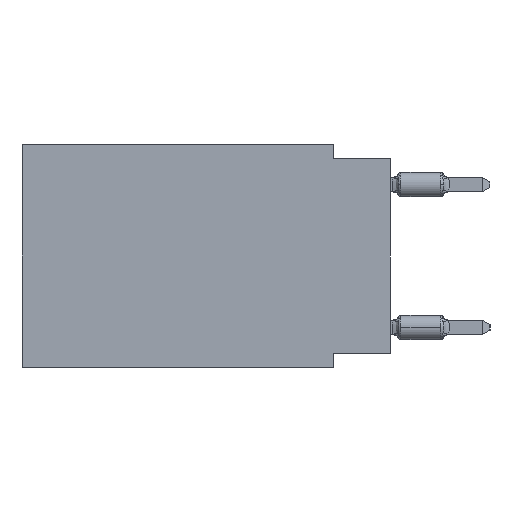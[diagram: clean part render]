
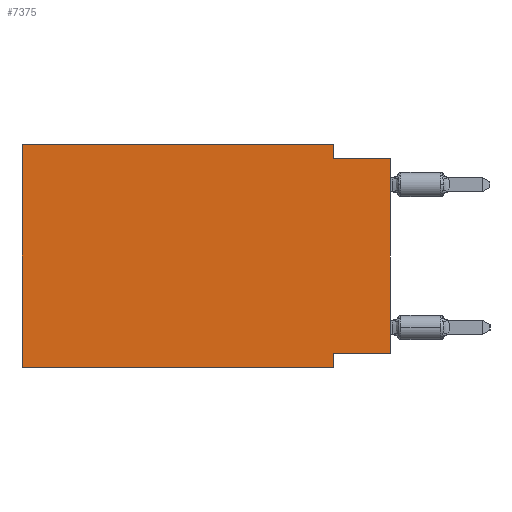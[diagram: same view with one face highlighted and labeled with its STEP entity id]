
A CAD part, left-side view. The second image highlights one B-rep face of the part: STEP entity #7375.
In plain terms, the highlighted planar face has unit normal (-1, 0, 0).
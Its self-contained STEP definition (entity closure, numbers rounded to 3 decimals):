
#169 = CARTESIAN_POINT ( 'NONE',  ( 0., 2.54, 0. ) ) ;
#2440 = ORIENTED_EDGE ( 'NONE', *, *, #37005, .T. ) ;
#3005 = VERTEX_POINT ( 'NONE', #38410 ) ;
#3457 = LINE ( 'NONE', #36537, #50990 ) ;
#3582 = LINE ( 'NONE', #32862, #7702 ) ;
#3731 = VECTOR ( 'NONE', #11823, 1000. ) ;
#4419 = VECTOR ( 'NONE', #9412, 1000. ) ;
#6550 = DIRECTION ( 'NONE',  ( 0., 0., 1. ) ) ;
#6747 = CARTESIAN_POINT ( 'NONE',  ( 0., 16.383, 0. ) ) ;
#7021 = ORIENTED_EDGE ( 'NONE', *, *, #34202, .T. ) ;
#7237 = DIRECTION ( 'NONE',  ( 0., -1., 0. ) ) ;
#7350 = CARTESIAN_POINT ( 'NONE',  ( 0., 16.383, 0. ) ) ;
#7375 = ADVANCED_FACE ( 'NONE', ( #44193 ), #24103, .F. ) ;
#7702 = VECTOR ( 'NONE', #44276, 1000. ) ;
#7764 = EDGE_CURVE ( 'NONE', #28013, #42736, #15905, .T. ) ;
#8222 = CARTESIAN_POINT ( 'NONE',  ( 0., 0., -9.271 ) ) ;
#9412 = DIRECTION ( 'NONE',  ( 0., -1., 0. ) ) ;
#10218 = CARTESIAN_POINT ( 'NONE',  ( 0., 2.54, -9.271 ) ) ;
#11292 = CARTESIAN_POINT ( 'NONE',  ( 0., 16.383, 0. ) ) ;
#11357 = DIRECTION ( 'NONE',  ( 0., 0., -1. ) ) ;
#11823 = DIRECTION ( 'NONE',  ( 0., -1., 0. ) ) ;
#14249 = LINE ( 'NONE', #37858, #24357 ) ;
#15905 = LINE ( 'NONE', #11292, #3731 ) ;
#16024 = EDGE_CURVE ( 'NONE', #24890, #28013, #16033, .T. ) ;
#16033 = LINE ( 'NONE', #7350, #24914 ) ;
#17414 = ORIENTED_EDGE ( 'NONE', *, *, #48316, .F. ) ;
#19610 = EDGE_CURVE ( 'NONE', #3005, #48276, #41993, .T. ) ;
#20754 = LINE ( 'NONE', #169, #43740 ) ;
#21306 = DIRECTION ( 'NONE',  ( 0., 1., 0. ) ) ;
#23754 = ORIENTED_EDGE ( 'NONE', *, *, #16024, .F. ) ;
#24103 = PLANE ( 'NONE',  #35739 ) ;
#24357 = VECTOR ( 'NONE', #21306, 1000. ) ;
#24890 = VERTEX_POINT ( 'NONE', #26294 ) ;
#24914 = VECTOR ( 'NONE', #6550, 1000. ) ;
#25377 = VERTEX_POINT ( 'NONE', #10218 ) ;
#26294 = CARTESIAN_POINT ( 'NONE',  ( 0., 16.383, -9.906 ) ) ;
#26539 = DIRECTION ( 'NONE',  ( 0., 0., 1. ) ) ;
#28013 = VERTEX_POINT ( 'NONE', #35635 ) ;
#29363 = VERTEX_POINT ( 'NONE', #8222 ) ;
#29427 = ORIENTED_EDGE ( 'NONE', *, *, #19610, .F. ) ;
#30350 = ORIENTED_EDGE ( 'NONE', *, *, #53325, .F. ) ;
#30877 = CARTESIAN_POINT ( 'NONE',  ( 0., 0., 0. ) ) ;
#32862 = CARTESIAN_POINT ( 'NONE',  ( 0., 2.54, -9.906 ) ) ;
#33227 = DIRECTION ( 'NONE',  ( 0., 0., -1. ) ) ;
#34202 = EDGE_CURVE ( 'NONE', #24890, #43339, #3457, .T. ) ;
#34960 = LINE ( 'NONE', #30877, #52023 ) ;
#35383 = EDGE_LOOP ( 'NONE', ( #2440, #29427, #17414, #42789, #23754, #7021, #30350, #47839 ) ) ;
#35635 = CARTESIAN_POINT ( 'NONE',  ( 0., 16.383, 0. ) ) ;
#35739 = AXIS2_PLACEMENT_3D ( 'NONE', #6747, #43925, #11357 ) ;
#36537 = CARTESIAN_POINT ( 'NONE',  ( 0., 16.383, -9.906 ) ) ;
#37005 = EDGE_CURVE ( 'NONE', #29363, #48276, #34960, .T. ) ;
#37018 = CARTESIAN_POINT ( 'NONE',  ( 0., 2.54, -9.906 ) ) ;
#37477 = CARTESIAN_POINT ( 'NONE',  ( 0., 2.54, 0. ) ) ;
#37858 = CARTESIAN_POINT ( 'NONE',  ( 0., 0., -9.271 ) ) ;
#37996 = EDGE_CURVE ( 'NONE', #29363, #25377, #14249, .T. ) ;
#38410 = CARTESIAN_POINT ( 'NONE',  ( 0., 2.54, -0.635 ) ) ;
#41993 = LINE ( 'NONE', #43062, #4419 ) ;
#42736 = VERTEX_POINT ( 'NONE', #37477 ) ;
#42789 = ORIENTED_EDGE ( 'NONE', *, *, #7764, .F. ) ;
#43062 = CARTESIAN_POINT ( 'NONE',  ( 0., 0., -0.635 ) ) ;
#43339 = VERTEX_POINT ( 'NONE', #37018 ) ;
#43740 = VECTOR ( 'NONE', #33227, 1000. ) ;
#43925 = DIRECTION ( 'NONE',  ( 1., 0., 0. ) ) ;
#44193 = FACE_OUTER_BOUND ( 'NONE', #35383, .T. ) ;
#44276 = DIRECTION ( 'NONE',  ( 0., 0., -1. ) ) ;
#45185 = CARTESIAN_POINT ( 'NONE',  ( 0., 0., -0.635 ) ) ;
#47839 = ORIENTED_EDGE ( 'NONE', *, *, #37996, .F. ) ;
#48276 = VERTEX_POINT ( 'NONE', #45185 ) ;
#48316 = EDGE_CURVE ( 'NONE', #42736, #3005, #20754, .T. ) ;
#50990 = VECTOR ( 'NONE', #7237, 1000. ) ;
#52023 = VECTOR ( 'NONE', #26539, 1000. ) ;
#53325 = EDGE_CURVE ( 'NONE', #25377, #43339, #3582, .T. ) ;
